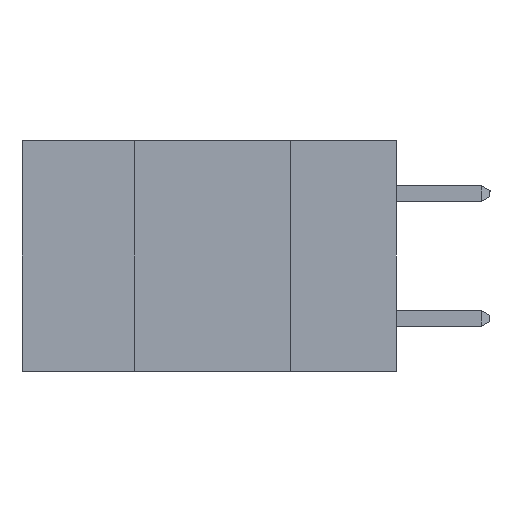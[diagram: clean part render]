
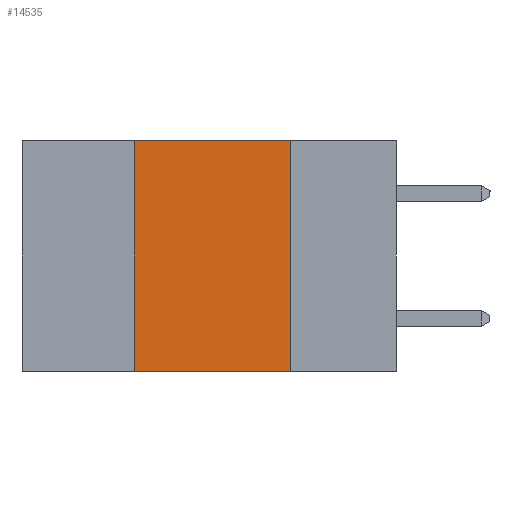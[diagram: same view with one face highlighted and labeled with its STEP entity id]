
A CAD part, left-side view. The second image highlights one B-rep face of the part: STEP entity #14535.
In plain terms, the highlighted planar face has unit normal (-1, 0, 0).
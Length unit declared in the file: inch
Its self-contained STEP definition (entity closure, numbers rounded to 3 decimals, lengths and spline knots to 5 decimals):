
#18 = EDGE_CURVE ( 'NONE', #2691, #8898, #9657, .T. ) ;
#2691 = VERTEX_POINT ( 'NONE', #7228 ) ;
#3261 = AXIS2_PLACEMENT_3D ( 'NONE', #6777, #10415, #14560 ) ;
#3279 = LINE ( 'NONE', #20669, #19792 ) ;
#4084 = DIRECTION ( 'NONE',  ( 0., 0., -1. ) ) ;
#4487 = DIRECTION ( 'NONE',  ( 0., 0., 1. ) ) ;
#6047 = VECTOR ( 'NONE', #17772, 39.37008 ) ;
#6777 = CARTESIAN_POINT ( 'NONE',  ( 0., 0.6, 0. ) ) ;
#7228 = CARTESIAN_POINT ( 'NONE',  ( 0., 0.17, 0. ) ) ;
#7380 = VECTOR ( 'NONE', #4084, 39.37008 ) ;
#7835 = CARTESIAN_POINT ( 'NONE',  ( 0., 0.42, 0. ) ) ;
#7908 = LINE ( 'NONE', #15933, #6047 ) ;
#8898 = VERTEX_POINT ( 'NONE', #17142 ) ;
#9657 = LINE ( 'NONE', #13545, #7380 ) ;
#9762 = EDGE_CURVE ( 'NONE', #14589, #8898, #7908, .T. ) ;
#10415 = DIRECTION ( 'NONE',  ( 1., 0., 0. ) ) ;
#12607 = PLANE ( 'NONE',  #3261 ) ;
#13545 = CARTESIAN_POINT ( 'NONE',  ( 0., 0.17, -0.37 ) ) ;
#13584 = EDGE_LOOP ( 'NONE', ( #14583, #20906, #18752, #20186 ) ) ;
#14535 = ADVANCED_FACE ( 'NONE', ( #18454 ), #12607, .F. ) ;
#14560 = DIRECTION ( 'NONE',  ( 0., 0., -1. ) ) ;
#14583 = ORIENTED_EDGE ( 'NONE', *, *, #18, .F. ) ;
#14589 = VERTEX_POINT ( 'NONE', #18592 ) ;
#14817 = DIRECTION ( 'NONE',  ( 0., -1., 0. ) ) ;
#15933 = CARTESIAN_POINT ( 'NONE',  ( 0., 0.6, -0.37 ) ) ;
#16783 = CARTESIAN_POINT ( 'NONE',  ( 0., 0.42, -0.37 ) ) ;
#17142 = CARTESIAN_POINT ( 'NONE',  ( 0., 0.17, -0.37 ) ) ;
#17636 = VECTOR ( 'NONE', #4487, 39.37008 ) ;
#17772 = DIRECTION ( 'NONE',  ( 0., -1., 0. ) ) ;
#18454 = FACE_OUTER_BOUND ( 'NONE', #13584, .T. ) ;
#18592 = CARTESIAN_POINT ( 'NONE',  ( 0., 0.42, -0.37 ) ) ;
#18752 = ORIENTED_EDGE ( 'NONE', *, *, #18772, .F. ) ;
#18772 = EDGE_CURVE ( 'NONE', #14589, #21989, #22126, .T. ) ;
#19792 = VECTOR ( 'NONE', #14817, 39.37008 ) ;
#20186 = ORIENTED_EDGE ( 'NONE', *, *, #9762, .T. ) ;
#20669 = CARTESIAN_POINT ( 'NONE',  ( 0., 0.6, 0. ) ) ;
#20906 = ORIENTED_EDGE ( 'NONE', *, *, #23690, .F. ) ;
#21989 = VERTEX_POINT ( 'NONE', #7835 ) ;
#22126 = LINE ( 'NONE', #16783, #17636 ) ;
#23690 = EDGE_CURVE ( 'NONE', #21989, #2691, #3279, .T. ) ;
